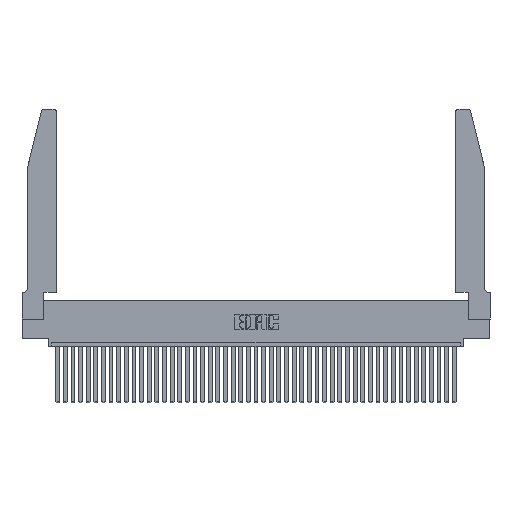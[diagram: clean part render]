
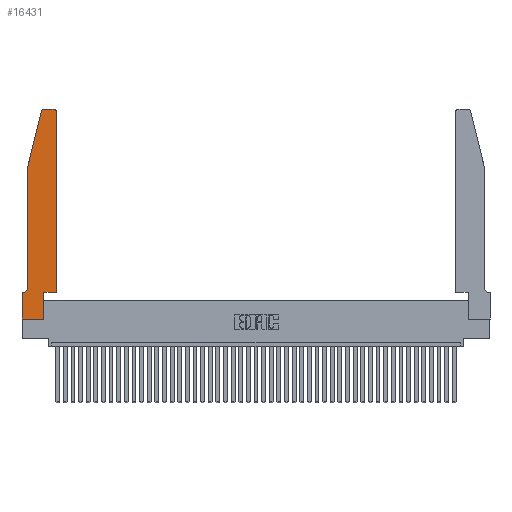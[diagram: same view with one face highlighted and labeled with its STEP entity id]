
A CAD part, top view. The second image highlights one B-rep face of the part: STEP entity #16431.
In plain terms, the highlighted planar face has unit normal (0, 0, 1).
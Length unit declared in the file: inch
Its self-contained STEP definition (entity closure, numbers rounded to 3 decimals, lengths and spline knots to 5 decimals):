
#32 = EDGE_CURVE ( 'NONE', #28097, #38828, #20482, .T. ) ;
#38 = EDGE_CURVE ( 'NONE', #253, #38577, #7396, .T. ) ;
#253 = VERTEX_POINT ( 'NONE', #24154 ) ;
#1088 = CARTESIAN_POINT ( 'NONE',  ( 0.4505, 2.72, 0.37 ) ) ;
#1319 = VERTEX_POINT ( 'NONE', #28440 ) ;
#1445 = CARTESIAN_POINT ( 'NONE',  ( 0.4505, 0.35, 0.37 ) ) ;
#1665 = ORIENTED_EDGE ( 'NONE', *, *, #32, .T. ) ;
#1923 = CARTESIAN_POINT ( 'NONE',  ( 0.4205, 2.75, 0.37 ) ) ;
#2345 = CARTESIAN_POINT ( 'NONE',  ( 0., 0.35, 0.37 ) ) ;
#2352 = CARTESIAN_POINT ( 'NONE',  ( 0.0055, 0.42, 0.37 ) ) ;
#2492 = DIRECTION ( 'NONE',  ( 0., 0., -1. ) ) ;
#3257 = ORIENTED_EDGE ( 'NONE', *, *, #6835, .T. ) ;
#3274 = VECTOR ( 'NONE', #17970, 39.37008 ) ;
#3369 = PLANE ( 'NONE',  #39200 ) ;
#4014 = LINE ( 'NONE', #19344, #24926 ) ;
#5508 = ORIENTED_EDGE ( 'NONE', *, *, #28117, .T. ) ;
#5621 = AXIS2_PLACEMENT_3D ( 'NONE', #5865, #16208, #26324 ) ;
#5865 = CARTESIAN_POINT ( 'NONE',  ( 0.284, 2.72, 0.37 ) ) ;
#6835 = EDGE_CURVE ( 'NONE', #38577, #40153, #19432, .T. ) ;
#6977 = ORIENTED_EDGE ( 'NONE', *, *, #38, .T. ) ;
#7396 = LINE ( 'NONE', #10838, #37631 ) ;
#9131 = CIRCLE ( 'NONE', #42818, 0.07 ) ;
#9175 = VERTEX_POINT ( 'NONE', #21678 ) ;
#9604 = CARTESIAN_POINT ( 'NONE',  ( 0.0755, 0.42, 0.37 ) ) ;
#9920 = ORIENTED_EDGE ( 'NONE', *, *, #39230, .T. ) ;
#9942 = VERTEX_POINT ( 'NONE', #25461 ) ;
#10326 = LINE ( 'NONE', #40092, #39007 ) ;
#10838 = CARTESIAN_POINT ( 'NONE',  ( 0.2865, 0.35, 0.37 ) ) ;
#11161 = CARTESIAN_POINT ( 'NONE',  ( 0.4505, 0.35, 0.37 ) ) ;
#11558 = VECTOR ( 'NONE', #22385, 39.37008 ) ;
#12915 = CARTESIAN_POINT ( 'NONE',  ( 0.0755, 2., 0.37 ) ) ;
#12984 = VERTEX_POINT ( 'NONE', #2345 ) ;
#13393 = EDGE_CURVE ( 'NONE', #1319, #9175, #20005, .T. ) ;
#13940 = ORIENTED_EDGE ( 'NONE', *, *, #16189, .T. ) ;
#13957 = ORIENTED_EDGE ( 'NONE', *, *, #17506, .T. ) ;
#14184 = ORIENTED_EDGE ( 'NONE', *, *, #16932, .T. ) ;
#14655 = VECTOR ( 'NONE', #25175, 39.37008 ) ;
#16189 = EDGE_CURVE ( 'NONE', #12984, #9942, #10326, .T. ) ;
#16208 = DIRECTION ( 'NONE',  ( 0., 0., 1. ) ) ;
#16431 = ADVANCED_FACE ( 'NONE', ( #37435 ), #3369, .T. ) ;
#16885 = EDGE_CURVE ( 'NONE', #38828, #29934, #9131, .T. ) ;
#16932 = EDGE_CURVE ( 'NONE', #9942, #253, #21135, .T. ) ;
#17506 = EDGE_CURVE ( 'NONE', #22068, #25507, #17892, .T. ) ;
#17892 = CIRCLE ( 'NONE', #26539, 0.03 ) ;
#17970 = DIRECTION ( 'NONE',  ( 0., -1., 0. ) ) ;
#18305 = CARTESIAN_POINT ( 'NONE',  ( 0.0755, 2., 0.37 ) ) ;
#18377 = VECTOR ( 'NONE', #32195, 39.37008 ) ;
#18509 = VECTOR ( 'NONE', #42148, 39.37008 ) ;
#18854 = CARTESIAN_POINT ( 'NONE',  ( 0., 0., 0.37 ) ) ;
#19010 = CARTESIAN_POINT ( 'NONE',  ( 0.0755, 0.35, 0.37 ) ) ;
#19344 = CARTESIAN_POINT ( 'NONE',  ( 0.2605, 2.75, 0.37 ) ) ;
#19432 = LINE ( 'NONE', #1445, #18377 ) ;
#20005 = CIRCLE ( 'NONE', #5621, 0.03 ) ;
#20482 = LINE ( 'NONE', #12915, #3274 ) ;
#20820 = EDGE_CURVE ( 'NONE', #40153, #22068, #25538, .T. ) ;
#21135 = LINE ( 'NONE', #18854, #18509 ) ;
#21678 = CARTESIAN_POINT ( 'NONE',  ( 0.25487, 2.72718, 0.37 ) ) ;
#21871 = ORIENTED_EDGE ( 'NONE', *, *, #13393, .T. ) ;
#22026 = LINE ( 'NONE', #19010, #11558 ) ;
#22068 = VERTEX_POINT ( 'NONE', #1088 ) ;
#22385 = DIRECTION ( 'NONE',  ( -1., 0., 0. ) ) ;
#22495 = DIRECTION ( 'NONE',  ( 1., 0., 0. ) ) ;
#22637 = DIRECTION ( 'NONE',  ( 0., 0., 1. ) ) ;
#22699 = DIRECTION ( 'NONE',  ( 0., 1., 0. ) ) ;
#23433 = VECTOR ( 'NONE', #37375, 39.37008 ) ;
#24154 = CARTESIAN_POINT ( 'NONE',  ( 0.2865, 0., 0.37 ) ) ;
#24926 = VECTOR ( 'NONE', #42196, 39.37008 ) ;
#25108 = EDGE_CURVE ( 'NONE', #29934, #12984, #22026, .T. ) ;
#25175 = DIRECTION ( 'NONE',  ( -0.239, -0.971, 0. ) ) ;
#25213 = EDGE_LOOP ( 'NONE', ( #5508, #21871, #9920, #1665, #25230, #32529, #13940, #14184, #6977, #3257, #39900, #13957 ) ) ;
#25230 = ORIENTED_EDGE ( 'NONE', *, *, #16885, .T. ) ;
#25461 = CARTESIAN_POINT ( 'NONE',  ( 0., 0., 0.37 ) ) ;
#25507 = VERTEX_POINT ( 'NONE', #1923 ) ;
#25538 = LINE ( 'NONE', #11161, #23433 ) ;
#26324 = DIRECTION ( 'NONE',  ( 1., 0., 0. ) ) ;
#26539 = AXIS2_PLACEMENT_3D ( 'NONE', #26835, #26687, #30443 ) ;
#26687 = DIRECTION ( 'NONE',  ( 0., 0., 1. ) ) ;
#26835 = CARTESIAN_POINT ( 'NONE',  ( 0.4205, 2.72, 0.37 ) ) ;
#28097 = VERTEX_POINT ( 'NONE', #29266 ) ;
#28117 = EDGE_CURVE ( 'NONE', #25507, #1319, #4014, .T. ) ;
#28424 = CARTESIAN_POINT ( 'NONE',  ( 0.0055, 0.35, 0.37 ) ) ;
#28440 = CARTESIAN_POINT ( 'NONE',  ( 0.284, 2.75, 0.37 ) ) ;
#29184 = DIRECTION ( 'NONE',  ( -1., 0., 0. ) ) ;
#29266 = CARTESIAN_POINT ( 'NONE',  ( 0.0755, 2., 0.37 ) ) ;
#29296 = LINE ( 'NONE', #18305, #14655 ) ;
#29322 = CARTESIAN_POINT ( 'NONE',  ( 0., 0.35, 0.37 ) ) ;
#29934 = VERTEX_POINT ( 'NONE', #28424 ) ;
#30186 = DIRECTION ( 'NONE',  ( 0., -1., 0. ) ) ;
#30443 = DIRECTION ( 'NONE',  ( 1., 0., 0. ) ) ;
#30462 = CARTESIAN_POINT ( 'NONE',  ( 0.2865, 0.35, 0.37 ) ) ;
#32195 = DIRECTION ( 'NONE',  ( 1., 0., 0. ) ) ;
#32529 = ORIENTED_EDGE ( 'NONE', *, *, #25108, .T. ) ;
#33379 = CARTESIAN_POINT ( 'NONE',  ( 0.4505, 0.35, 0.37 ) ) ;
#37375 = DIRECTION ( 'NONE',  ( 0., 1., 0. ) ) ;
#37435 = FACE_OUTER_BOUND ( 'NONE', #25213, .T. ) ;
#37631 = VECTOR ( 'NONE', #22699, 39.37008 ) ;
#38577 = VERTEX_POINT ( 'NONE', #30462 ) ;
#38828 = VERTEX_POINT ( 'NONE', #9604 ) ;
#39007 = VECTOR ( 'NONE', #30186, 39.37008 ) ;
#39200 = AXIS2_PLACEMENT_3D ( 'NONE', #29322, #22637, #22495 ) ;
#39230 = EDGE_CURVE ( 'NONE', #9175, #28097, #29296, .T. ) ;
#39900 = ORIENTED_EDGE ( 'NONE', *, *, #20820, .T. ) ;
#40092 = CARTESIAN_POINT ( 'NONE',  ( 0., 0., 0.37 ) ) ;
#40153 = VERTEX_POINT ( 'NONE', #33379 ) ;
#42148 = DIRECTION ( 'NONE',  ( 1., 0., 0. ) ) ;
#42196 = DIRECTION ( 'NONE',  ( -1., 0., 0. ) ) ;
#42818 = AXIS2_PLACEMENT_3D ( 'NONE', #2352, #2492, #29184 ) ;
